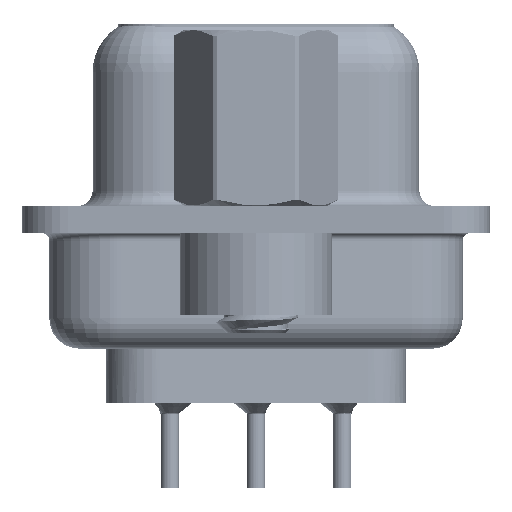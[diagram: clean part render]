
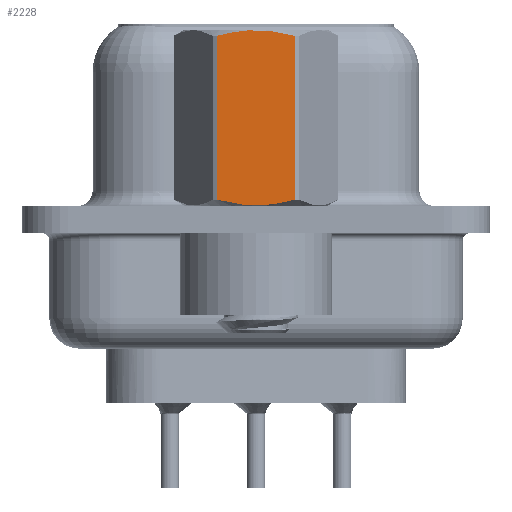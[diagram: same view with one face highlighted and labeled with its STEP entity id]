
A CAD part, left-side view. The second image highlights one B-rep face of the part: STEP entity #2228.
In plain terms, the highlighted planar face has unit normal (-1, 0, 0).
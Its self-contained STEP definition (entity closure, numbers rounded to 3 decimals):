
#651 = EDGE_CURVE ( 'NONE', #32095, #43258, #19687, .T. ) ;
#653 = CARTESIAN_POINT ( 'NONE',  ( -2.381, 1.273, 3.792 ) ) ;
#1933 = CARTESIAN_POINT ( 'NONE',  ( -2.381, 0.215, 0.468 ) ) ;
#2087 = CARTESIAN_POINT ( 'NONE',  ( -2.381, -0.215, 0.468 ) ) ;
#2228 = ADVANCED_FACE ( 'NONE', ( #17829 ), #16986, .T. ) ;
#5037 = CARTESIAN_POINT ( 'NONE',  ( -2.381, 0.853, 0.549 ) ) ;
#5290 = DIRECTION ( 'NONE',  ( 0., -1., 0. ) ) ;
#5334 = DIRECTION ( 'NONE',  ( -1., 0., 0. ) ) ;
#5343 = CARTESIAN_POINT ( 'NONE',  ( -2.381, 1.375, -3.75 ) ) ;
#5984 = ORIENTED_EDGE ( 'NONE', *, *, #6796, .T. ) ;
#6581 = CARTESIAN_POINT ( 'NONE',  ( -2.381, -1.273, 0.652 ) ) ;
#6796 = EDGE_CURVE ( 'NONE', #43258, #40360, #38281, .T. ) ;
#6798 = CARTESIAN_POINT ( 'NONE',  ( -2.381, -0.432, 0.485 ) ) ;
#6897 = CARTESIAN_POINT ( 'NONE',  ( -2.381, -1.273, 6.048 ) ) ;
#7337 = CARTESIAN_POINT ( 'NONE',  ( -2.381, 1.273, 0.652 ) ) ;
#8504 = LINE ( 'NONE', #653, #26547 ) ;
#9934 = CARTESIAN_POINT ( 'NONE',  ( -2.381, -0.858, 0.55 ) ) ;
#10185 = ORIENTED_EDGE ( 'NONE', *, *, #651, .T. ) ;
#10527 = CARTESIAN_POINT ( 'NONE',  ( -2.381, -0.432, 6.215 ) ) ;
#10911 = CARTESIAN_POINT ( 'NONE',  ( -2.381, -1.066, 0.596 ) ) ;
#11601 = DIRECTION ( 'NONE',  ( 0., 0., -1. ) ) ;
#14149 = CARTESIAN_POINT ( 'NONE',  ( -2.381, 0.215, 6.232 ) ) ;
#16004 = ORIENTED_EDGE ( 'NONE', *, *, #40534, .T. ) ;
#16199 = CARTESIAN_POINT ( 'NONE',  ( -2.381, -1.273, 3.792 ) ) ;
#16986 = PLANE ( 'NONE',  #36513 ) ;
#17507 = CARTESIAN_POINT ( 'NONE',  ( -2.381, -0.858, 6.15 ) ) ;
#17827 = CARTESIAN_POINT ( 'NONE',  ( -2.381, 0.853, 6.151 ) ) ;
#17829 = FACE_OUTER_BOUND ( 'NONE', #23528, .T. ) ;
#19292 = VECTOR ( 'NONE', #41347, 1000. ) ;
#19687 = B_SPLINE_CURVE_WITH_KNOTS ( 'NONE', 3,
 ( #37438, #37492, #5037, #39682, #1933, #2087, #6798, #9934, #10911, #6581 ),
 .UNSPECIFIED., .F., .F.,
 ( 4, 2, 2, 2, 4 ),
 ( 0.003, 0.003, 0.004, 0.004, 0.005 ),
 .UNSPECIFIED. ) ;
#21438 = CARTESIAN_POINT ( 'NONE',  ( -2.381, 1.273, 6.048 ) ) ;
#22811 = EDGE_CURVE ( 'NONE', #40360, #25979, #34257, .T. ) ;
#23528 = EDGE_LOOP ( 'NONE', ( #10185, #5984, #29703, #16004 ) ) ;
#25764 = CARTESIAN_POINT ( 'NONE',  ( -2.381, -1.273, 0.652 ) ) ;
#25979 = VERTEX_POINT ( 'NONE', #39943 ) ;
#26547 = VECTOR ( 'NONE', #11601, 1000. ) ;
#28450 = CARTESIAN_POINT ( 'NONE',  ( -2.381, -1.066, 6.104 ) ) ;
#29703 = ORIENTED_EDGE ( 'NONE', *, *, #22811, .T. ) ;
#31558 = CARTESIAN_POINT ( 'NONE',  ( -2.381, -1.273, 6.048 ) ) ;
#32095 = VERTEX_POINT ( 'NONE', #7337 ) ;
#34257 = B_SPLINE_CURVE_WITH_KNOTS ( 'NONE', 3,
 ( #6897, #28450, #17507, #10527, #35642, #14149, #39204, #17827, #42824, #21438 ),
 .UNSPECIFIED., .F., .F.,
 ( 4, 2, 2, 2, 4 ),
 ( 0.001, 0.002, 0.002, 0.003, 0.004 ),
 .UNSPECIFIED. ) ;
#35642 = CARTESIAN_POINT ( 'NONE',  ( -2.381, -0.215, 6.232 ) ) ;
#36513 = AXIS2_PLACEMENT_3D ( 'NONE', #5343, #5334, #5290 ) ;
#37438 = CARTESIAN_POINT ( 'NONE',  ( -2.381, 1.273, 0.652 ) ) ;
#37492 = CARTESIAN_POINT ( 'NONE',  ( -2.381, 1.065, 0.596 ) ) ;
#38281 = LINE ( 'NONE', #16199, #19292 ) ;
#39204 = CARTESIAN_POINT ( 'NONE',  ( -2.381, 0.428, 6.215 ) ) ;
#39682 = CARTESIAN_POINT ( 'NONE',  ( -2.381, 0.428, 0.485 ) ) ;
#39943 = CARTESIAN_POINT ( 'NONE',  ( -2.381, 1.273, 6.048 ) ) ;
#40360 = VERTEX_POINT ( 'NONE', #31558 ) ;
#40534 = EDGE_CURVE ( 'NONE', #25979, #32095, #8504, .T. ) ;
#41347 = DIRECTION ( 'NONE',  ( 0., 0., 1. ) ) ;
#42824 = CARTESIAN_POINT ( 'NONE',  ( -2.381, 1.065, 6.104 ) ) ;
#43258 = VERTEX_POINT ( 'NONE', #25764 ) ;
